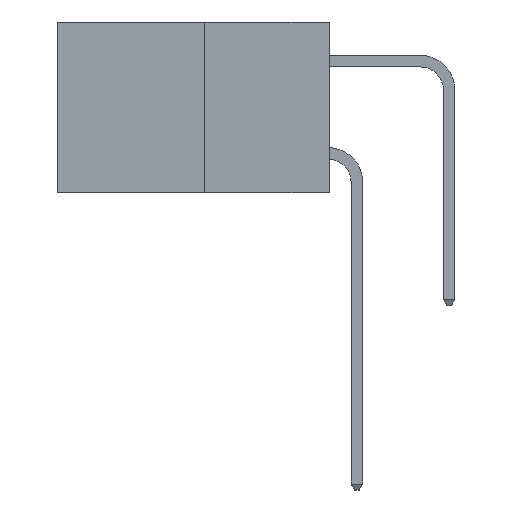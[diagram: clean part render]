
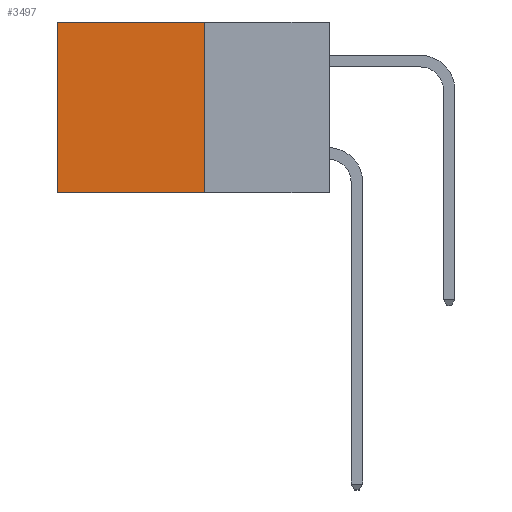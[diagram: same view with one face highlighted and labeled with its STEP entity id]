
A CAD part, left-side view. The second image highlights one B-rep face of the part: STEP entity #3497.
In plain terms, the highlighted planar face has unit normal (-1, 0, 0).
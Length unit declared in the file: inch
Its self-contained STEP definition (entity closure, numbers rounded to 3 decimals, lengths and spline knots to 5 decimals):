
#119 = CARTESIAN_POINT ( 'NONE',  ( 0.277, 0.59, -0.37 ) ) ;
#606 = VERTEX_POINT ( 'NONE', #15251 ) ;
#695 = ORIENTED_EDGE ( 'NONE', *, *, #14463, .T. ) ;
#991 = VECTOR ( 'NONE', #8277, 39.37008 ) ;
#1236 = CARTESIAN_POINT ( 'NONE',  ( 0.277, 0.27, 0. ) ) ;
#1266 = ORIENTED_EDGE ( 'NONE', *, *, #14057, .F. ) ;
#1860 = CARTESIAN_POINT ( 'NONE',  ( 0.277, 0.59, 0. ) ) ;
#2026 = DIRECTION ( 'NONE',  ( 0., 0., -1. ) ) ;
#3497 = ADVANCED_FACE ( 'NONE', ( #17742 ), #7932, .F. ) ;
#3630 = VERTEX_POINT ( 'NONE', #1236 ) ;
#4652 = VECTOR ( 'NONE', #5541, 39.37008 ) ;
#5306 = EDGE_LOOP ( 'NONE', ( #695, #14625, #1266, #19491 ) ) ;
#5541 = DIRECTION ( 'NONE',  ( 0., 0., -1. ) ) ;
#6822 = VECTOR ( 'NONE', #8709, 39.37008 ) ;
#6993 = CARTESIAN_POINT ( 'NONE',  ( 0.277, 0.27, 0. ) ) ;
#7862 = CARTESIAN_POINT ( 'NONE',  ( 0.277, 0.27, -0.37 ) ) ;
#7932 = PLANE ( 'NONE',  #17184 ) ;
#8099 = CARTESIAN_POINT ( 'NONE',  ( 0.277, 0.27, -0.37 ) ) ;
#8173 = DIRECTION ( 'NONE',  ( 0., 1., 0. ) ) ;
#8277 = DIRECTION ( 'NONE',  ( 0., 0., -1. ) ) ;
#8709 = DIRECTION ( 'NONE',  ( 0., 1., 0. ) ) ;
#9220 = LINE ( 'NONE', #119, #4652 ) ;
#9562 = VERTEX_POINT ( 'NONE', #1860 ) ;
#11353 = LINE ( 'NONE', #6993, #6822 ) ;
#11568 = CARTESIAN_POINT ( 'NONE',  ( 0.277, 0.27, -0.37 ) ) ;
#12846 = EDGE_CURVE ( 'NONE', #14012, #606, #13577, .T. ) ;
#13577 = LINE ( 'NONE', #8099, #17980 ) ;
#14012 = VERTEX_POINT ( 'NONE', #11568 ) ;
#14057 = EDGE_CURVE ( 'NONE', #3630, #14012, #21954, .T. ) ;
#14364 = EDGE_CURVE ( 'NONE', #3630, #9562, #11353, .T. ) ;
#14463 = EDGE_CURVE ( 'NONE', #9562, #606, #9220, .T. ) ;
#14625 = ORIENTED_EDGE ( 'NONE', *, *, #12846, .F. ) ;
#15251 = CARTESIAN_POINT ( 'NONE',  ( 0.277, 0.59, -0.37 ) ) ;
#15793 = DIRECTION ( 'NONE',  ( 1., 0., 0. ) ) ;
#17184 = AXIS2_PLACEMENT_3D ( 'NONE', #7862, #15793, #2026 ) ;
#17742 = FACE_OUTER_BOUND ( 'NONE', #5306, .T. ) ;
#17980 = VECTOR ( 'NONE', #8173, 39.37008 ) ;
#18402 = CARTESIAN_POINT ( 'NONE',  ( 0.277, 0.27, -0.37 ) ) ;
#19491 = ORIENTED_EDGE ( 'NONE', *, *, #14364, .T. ) ;
#21954 = LINE ( 'NONE', #18402, #991 ) ;
